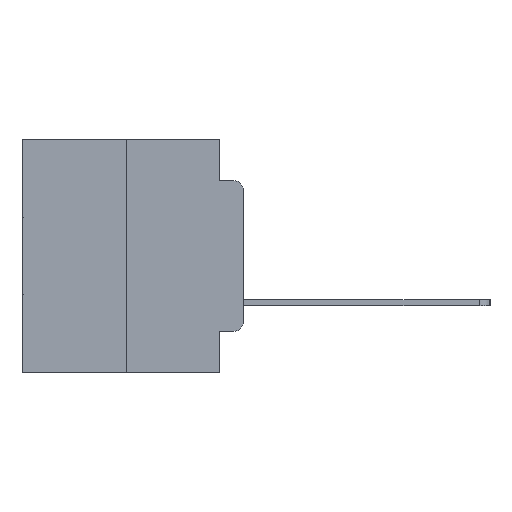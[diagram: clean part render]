
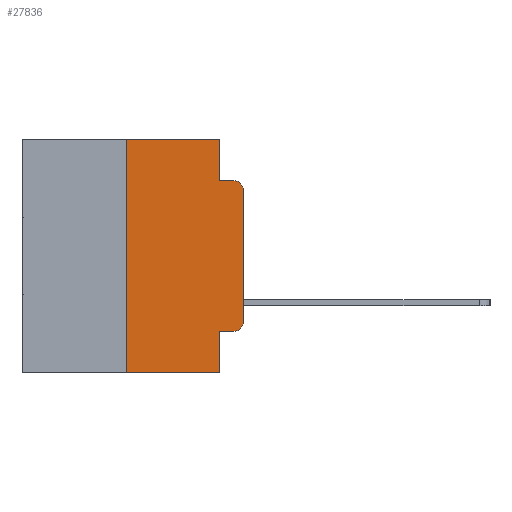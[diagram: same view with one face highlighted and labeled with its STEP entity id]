
A CAD part, left-side view. The second image highlights one B-rep face of the part: STEP entity #27836.
In plain terms, the highlighted planar face has unit normal (-1, 0, 0).
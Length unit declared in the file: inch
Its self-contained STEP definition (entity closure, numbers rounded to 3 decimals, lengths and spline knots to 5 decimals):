
#387 = ORIENTED_EDGE ( 'NONE', *, *, #14486, .F. ) ;
#639 = CARTESIAN_POINT ( 'NONE',  ( 0., 0.02, -0.4115 ) ) ;
#1207 = VERTEX_POINT ( 'NONE', #6710 ) ;
#1956 = CARTESIAN_POINT ( 'NONE',  ( 0., 0.473, 0. ) ) ;
#1985 = CARTESIAN_POINT ( 'NONE',  ( 0., 0.051, -0.4115 ) ) ;
#4026 = EDGE_CURVE ( 'NONE', #24782, #11295, #16418, .T. ) ;
#4300 = ORIENTED_EDGE ( 'NONE', *, *, #16045, .T. ) ;
#4723 = CARTESIAN_POINT ( 'NONE',  ( 0., 0.02, -0.1085 ) ) ;
#5695 = ORIENTED_EDGE ( 'NONE', *, *, #6486, .T. ) ;
#5774 = DIRECTION ( 'NONE',  ( 0., 0., -1. ) ) ;
#6220 = CARTESIAN_POINT ( 'NONE',  ( 0., 0.051, -0.5 ) ) ;
#6458 = CARTESIAN_POINT ( 'NONE',  ( 0., 0.051, -0.0885 ) ) ;
#6486 = EDGE_CURVE ( 'NONE', #24225, #1207, #11451, .T. ) ;
#6495 = DIRECTION ( 'NONE',  ( 0., 0., -1. ) ) ;
#6710 = CARTESIAN_POINT ( 'NONE',  ( 0., 0., -0.1085 ) ) ;
#6720 = VECTOR ( 'NONE', #12552, 39.37008 ) ;
#7022 = DIRECTION ( 'NONE',  ( 0., 0., -1. ) ) ;
#7228 = EDGE_CURVE ( 'NONE', #8175, #16317, #10373, .T. ) ;
#7421 = VECTOR ( 'NONE', #27551, 39.37008 ) ;
#8133 = LINE ( 'NONE', #16756, #7421 ) ;
#8175 = VERTEX_POINT ( 'NONE', #12448 ) ;
#8182 = EDGE_CURVE ( 'NONE', #16961, #17993, #12676, .T. ) ;
#8890 = CARTESIAN_POINT ( 'NONE',  ( 0., 0.051, 0. ) ) ;
#9079 = LINE ( 'NONE', #18186, #13585 ) ;
#9686 = VECTOR ( 'NONE', #11115, 39.37008 ) ;
#10050 = EDGE_CURVE ( 'NONE', #8175, #13202, #20005, .T. ) ;
#10362 = CARTESIAN_POINT ( 'NONE',  ( 0., 0.473, 0. ) ) ;
#10373 = LINE ( 'NONE', #8890, #9686 ) ;
#10570 = VECTOR ( 'NONE', #5774, 39.37008 ) ;
#10869 = DIRECTION ( 'NONE',  ( 0., 0., 1. ) ) ;
#11115 = DIRECTION ( 'NONE',  ( 0., 0., -1. ) ) ;
#11162 = FACE_OUTER_BOUND ( 'NONE', #13484, .T. ) ;
#11295 = VERTEX_POINT ( 'NONE', #6458 ) ;
#11451 = LINE ( 'NONE', #13109, #22324 ) ;
#12371 = ORIENTED_EDGE ( 'NONE', *, *, #4026, .F. ) ;
#12391 = ORIENTED_EDGE ( 'NONE', *, *, #7228, .F. ) ;
#12448 = CARTESIAN_POINT ( 'NONE',  ( 0., 0.051, -0.4115 ) ) ;
#12552 = DIRECTION ( 'NONE',  ( 0., 0., 1. ) ) ;
#12676 = LINE ( 'NONE', #27610, #6720 ) ;
#13109 = CARTESIAN_POINT ( 'NONE',  ( 0., 0., 0. ) ) ;
#13166 = AXIS2_PLACEMENT_3D ( 'NONE', #13301, #28302, #15490 ) ;
#13202 = VERTEX_POINT ( 'NONE', #639 ) ;
#13234 = LINE ( 'NONE', #10362, #18322 ) ;
#13301 = CARTESIAN_POINT ( 'NONE',  ( 0., 0.02, -0.3915 ) ) ;
#13484 = EDGE_LOOP ( 'NONE', ( #5695, #17469, #387, #12371, #25211, #19850, #4300, #12391, #19528, #14441 ) ) ;
#13502 = CIRCLE ( 'NONE', #13166, 0.02 ) ;
#13585 = VECTOR ( 'NONE', #24581, 39.37008 ) ;
#14257 = VECTOR ( 'NONE', #24034, 39.37008 ) ;
#14441 = ORIENTED_EDGE ( 'NONE', *, *, #17980, .T. ) ;
#14486 = EDGE_CURVE ( 'NONE', #11295, #19579, #8133, .T. ) ;
#14639 = CARTESIAN_POINT ( 'NONE',  ( 0., 0.051, 0. ) ) ;
#15306 = CARTESIAN_POINT ( 'NONE',  ( 0., 0.25, -0.5 ) ) ;
#15490 = DIRECTION ( 'NONE',  ( 0., 0., -1. ) ) ;
#15952 = EDGE_CURVE ( 'NONE', #1207, #19579, #16313, .T. ) ;
#16045 = EDGE_CURVE ( 'NONE', #16961, #16317, #9079, .T. ) ;
#16313 = CIRCLE ( 'NONE', #24175, 0.02 ) ;
#16317 = VERTEX_POINT ( 'NONE', #6220 ) ;
#16418 = LINE ( 'NONE', #14639, #10570 ) ;
#16756 = CARTESIAN_POINT ( 'NONE',  ( 0., 0.051, -0.0885 ) ) ;
#16961 = VERTEX_POINT ( 'NONE', #15306 ) ;
#17469 = ORIENTED_EDGE ( 'NONE', *, *, #15952, .T. ) ;
#17501 = PLANE ( 'NONE',  #23053 ) ;
#17980 = EDGE_CURVE ( 'NONE', #13202, #24225, #13502, .T. ) ;
#17993 = VERTEX_POINT ( 'NONE', #26230 ) ;
#18186 = CARTESIAN_POINT ( 'NONE',  ( 0., 0.473, -0.5 ) ) ;
#18322 = VECTOR ( 'NONE', #27682, 39.37008 ) ;
#19528 = ORIENTED_EDGE ( 'NONE', *, *, #10050, .T. ) ;
#19579 = VERTEX_POINT ( 'NONE', #25288 ) ;
#19671 = DIRECTION ( 'NONE',  ( 1., 0., 0. ) ) ;
#19850 = ORIENTED_EDGE ( 'NONE', *, *, #8182, .F. ) ;
#20005 = LINE ( 'NONE', #1985, #14257 ) ;
#20165 = DIRECTION ( 'NONE',  ( -1., 0., 0. ) ) ;
#22324 = VECTOR ( 'NONE', #10869, 39.37008 ) ;
#22745 = CARTESIAN_POINT ( 'NONE',  ( 0., 0., -0.3915 ) ) ;
#23053 = AXIS2_PLACEMENT_3D ( 'NONE', #1956, #19671, #6495 ) ;
#24034 = DIRECTION ( 'NONE',  ( 0., -1., 0. ) ) ;
#24175 = AXIS2_PLACEMENT_3D ( 'NONE', #4723, #20165, #7022 ) ;
#24225 = VERTEX_POINT ( 'NONE', #22745 ) ;
#24409 = EDGE_CURVE ( 'NONE', #17993, #24782, #13234, .T. ) ;
#24581 = DIRECTION ( 'NONE',  ( 0., -1., 0. ) ) ;
#24779 = CARTESIAN_POINT ( 'NONE',  ( 0., 0.051, 0. ) ) ;
#24782 = VERTEX_POINT ( 'NONE', #24779 ) ;
#25211 = ORIENTED_EDGE ( 'NONE', *, *, #24409, .F. ) ;
#25288 = CARTESIAN_POINT ( 'NONE',  ( 0., 0.02, -0.0885 ) ) ;
#26230 = CARTESIAN_POINT ( 'NONE',  ( 0., 0.25, 0. ) ) ;
#27551 = DIRECTION ( 'NONE',  ( 0., -1., 0. ) ) ;
#27610 = CARTESIAN_POINT ( 'NONE',  ( 0., 0.25, 0. ) ) ;
#27682 = DIRECTION ( 'NONE',  ( 0., -1., 0. ) ) ;
#27836 = ADVANCED_FACE ( 'NONE', ( #11162 ), #17501, .F. ) ;
#28302 = DIRECTION ( 'NONE',  ( -1., 0., 0. ) ) ;
